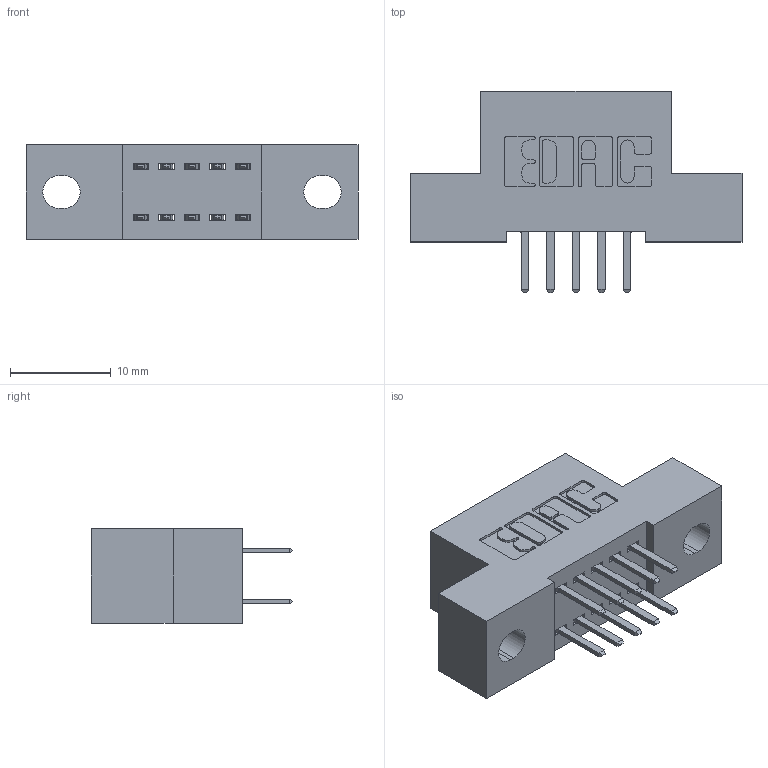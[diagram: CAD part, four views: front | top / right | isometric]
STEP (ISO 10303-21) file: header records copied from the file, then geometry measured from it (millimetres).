
FILE_DESCRIPTION (( 'STEP AP203' ), '1' );
FILE_NAME ('342-010-520-202.STEP', '2019-10-01T13:44:43', ( '' ), ( '' ), 'SwSTEP 2.0', 'SolidWorks 2016', '' );
FILE_SCHEMA (( 'CONFIG_CONTROL_DESIGN' ));
Length unit declared in the file: inch
Products named in the file (3): 342 Part_.128 Slot; 345-292-001_345-293-120; 342-010-520-202
Assembly tree (11 placements, depth 2):
  342-010-520-202
    342 Part_.128 Slot
    345-292-001_345-293-120  x10
Bounding box: 33.02 x 20.02 x 9.4 mm (x, y, z)
Volume: 2735.2 mm3; surface area: 3289.6 mm2
Topology: 11 solids, 11 shells, 674 faces, 1941 edges, 1266 vertices
Faces by surface type: plane 450, cylinder 224
Entity records: 8119 total; most frequent: CARTESIAN_POINT 1402, ORIENTED_EDGE 1326, DIRECTION 1251, EDGE_CURVE 663, VECTOR 531, LINE 531, VERTEX_POINT 438, AXIS2_PLACEMENT_3D 360
